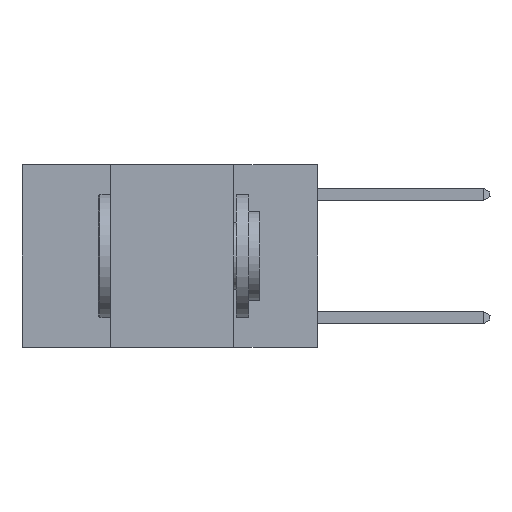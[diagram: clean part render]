
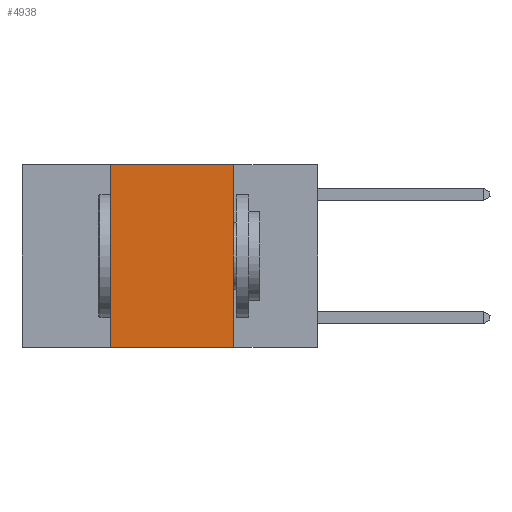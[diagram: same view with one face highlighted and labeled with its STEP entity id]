
A CAD part, left-side view. The second image highlights one B-rep face of the part: STEP entity #4938.
In plain terms, the highlighted planar face has unit normal (-1, 0, 0).
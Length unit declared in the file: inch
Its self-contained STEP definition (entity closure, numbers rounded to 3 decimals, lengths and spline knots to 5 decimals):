
#369 = VERTEX_POINT ( 'NONE', #3006 ) ;
#964 = CARTESIAN_POINT ( 'NONE',  ( 0., 0.42, 0. ) ) ;
#1261 = VERTEX_POINT ( 'NONE', #17274 ) ;
#1839 = VECTOR ( 'NONE', #17208, 39.37008 ) ;
#3006 = CARTESIAN_POINT ( 'NONE',  ( 0., 0.17, 0. ) ) ;
#3168 = LINE ( 'NONE', #8287, #12953 ) ;
#3469 = CARTESIAN_POINT ( 'NONE',  ( 0., 0.17, -0.37 ) ) ;
#3628 = VERTEX_POINT ( 'NONE', #3469 ) ;
#3698 = CARTESIAN_POINT ( 'NONE',  ( 0., 0.6, 0. ) ) ;
#4938 = ADVANCED_FACE ( 'NONE', ( #12267 ), #15381, .F. ) ;
#6394 = DIRECTION ( 'NONE',  ( 0., 0., -1. ) ) ;
#6519 = VECTOR ( 'NONE', #20161, 39.37008 ) ;
#6695 = DIRECTION ( 'NONE',  ( 0., 0., -1. ) ) ;
#7550 = ORIENTED_EDGE ( 'NONE', *, *, #12092, .T. ) ;
#8287 = CARTESIAN_POINT ( 'NONE',  ( 0., 0.17, 0. ) ) ;
#9397 = CARTESIAN_POINT ( 'NONE',  ( 0., 0.6, 0. ) ) ;
#10099 = EDGE_LOOP ( 'NONE', ( #11109, #20292, #13857, #7550 ) ) ;
#10439 = CARTESIAN_POINT ( 'NONE',  ( 0., 0.6, -0.37 ) ) ;
#10467 = DIRECTION ( 'NONE',  ( 1., 0., 0. ) ) ;
#11109 = ORIENTED_EDGE ( 'NONE', *, *, #16936, .F. ) ;
#12092 = EDGE_CURVE ( 'NONE', #1261, #3628, #12669, .T. ) ;
#12267 = FACE_OUTER_BOUND ( 'NONE', #10099, .T. ) ;
#12669 = LINE ( 'NONE', #10439, #1839 ) ;
#12953 = VECTOR ( 'NONE', #6394, 39.37008 ) ;
#13857 = ORIENTED_EDGE ( 'NONE', *, *, #16735, .F. ) ;
#15381 = PLANE ( 'NONE',  #17979 ) ;
#15812 = CARTESIAN_POINT ( 'NONE',  ( 0., 0.42, 0. ) ) ;
#16070 = LINE ( 'NONE', #9397, #6519 ) ;
#16735 = EDGE_CURVE ( 'NONE', #1261, #19796, #19294, .T. ) ;
#16825 = EDGE_CURVE ( 'NONE', #19796, #369, #16070, .T. ) ;
#16936 = EDGE_CURVE ( 'NONE', #369, #3628, #3168, .T. ) ;
#17208 = DIRECTION ( 'NONE',  ( 0., -1., 0. ) ) ;
#17274 = CARTESIAN_POINT ( 'NONE',  ( 0., 0.42, -0.37 ) ) ;
#17979 = AXIS2_PLACEMENT_3D ( 'NONE', #3698, #10467, #6695 ) ;
#19294 = LINE ( 'NONE', #964, #21773 ) ;
#19796 = VERTEX_POINT ( 'NONE', #15812 ) ;
#20161 = DIRECTION ( 'NONE',  ( 0., -1., 0. ) ) ;
#20292 = ORIENTED_EDGE ( 'NONE', *, *, #16825, .F. ) ;
#20949 = DIRECTION ( 'NONE',  ( 0., 0., 1. ) ) ;
#21773 = VECTOR ( 'NONE', #20949, 39.37008 ) ;
